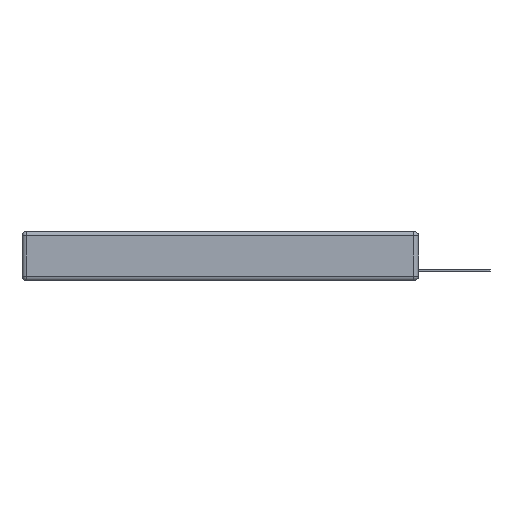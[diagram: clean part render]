
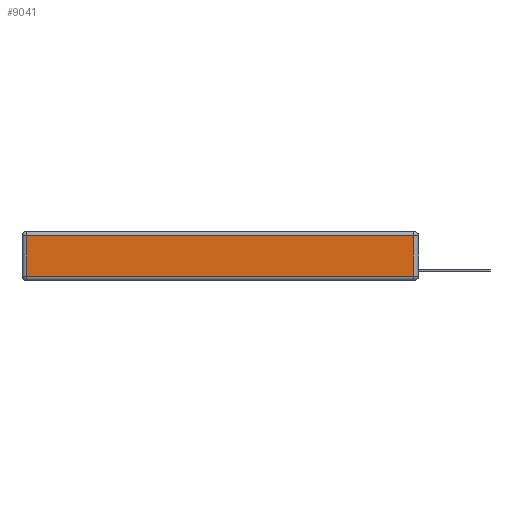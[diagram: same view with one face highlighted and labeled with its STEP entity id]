
A CAD part, left-side view. The second image highlights one B-rep face of the part: STEP entity #9041.
In plain terms, the highlighted planar face has unit normal (-1, 0, 0).
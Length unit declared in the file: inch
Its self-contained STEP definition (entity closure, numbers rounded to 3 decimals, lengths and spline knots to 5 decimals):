
#232 = EDGE_CURVE ( 'NONE', #12950, #11851, #2485, .T. ) ;
#245 = ORIENTED_EDGE ( 'NONE', *, *, #8034, .T. ) ;
#1006 = ORIENTED_EDGE ( 'NONE', *, *, #4992, .T. ) ;
#1263 = LINE ( 'NONE', #5545, #15086 ) ;
#1638 = DIRECTION ( 'NONE',  ( 0., 0., 1. ) ) ;
#2485 = LINE ( 'NONE', #7924, #13206 ) ;
#2680 = CARTESIAN_POINT ( 'NONE',  ( 0., 0.03, -0.313 ) ) ;
#3599 = VECTOR ( 'NONE', #1638, 39.37008 ) ;
#3632 = CARTESIAN_POINT ( 'NONE',  ( 0., 2.72, -0.03 ) ) ;
#4244 = CARTESIAN_POINT ( 'NONE',  ( 0., 2.72, -0.313 ) ) ;
#4803 = LINE ( 'NONE', #10966, #12752 ) ;
#4992 = EDGE_CURVE ( 'NONE', #8813, #12157, #4803, .T. ) ;
#4999 = CARTESIAN_POINT ( 'NONE',  ( 0., 0.03, -0.343 ) ) ;
#5394 = CARTESIAN_POINT ( 'NONE',  ( 0., 0.03, -0.03 ) ) ;
#5545 = CARTESIAN_POINT ( 'NONE',  ( 0., 2.72, -0.343 ) ) ;
#5698 = PLANE ( 'NONE',  #11499 ) ;
#5836 = LINE ( 'NONE', #4999, #3599 ) ;
#6877 = CARTESIAN_POINT ( 'NONE',  ( 0., 0., -0.343 ) ) ;
#7924 = CARTESIAN_POINT ( 'NONE',  ( 0., 2.75, -0.03 ) ) ;
#8034 = EDGE_CURVE ( 'NONE', #12157, #12950, #5836, .T. ) ;
#8718 = FACE_OUTER_BOUND ( 'NONE', #10525, .T. ) ;
#8813 = VERTEX_POINT ( 'NONE', #4244 ) ;
#9041 = ADVANCED_FACE ( 'NONE', ( #8718 ), #5698, .T. ) ;
#10252 = DIRECTION ( 'NONE',  ( 0., 0., -1. ) ) ;
#10482 = DIRECTION ( 'NONE',  ( 0., 0., 1. ) ) ;
#10525 = EDGE_LOOP ( 'NONE', ( #1006, #245, #13417, #14843 ) ) ;
#10966 = CARTESIAN_POINT ( 'NONE',  ( 0., 0., -0.313 ) ) ;
#11499 = AXIS2_PLACEMENT_3D ( 'NONE', #6877, #11743, #10482 ) ;
#11743 = DIRECTION ( 'NONE',  ( -1., 0., 0. ) ) ;
#11851 = VERTEX_POINT ( 'NONE', #3632 ) ;
#12157 = VERTEX_POINT ( 'NONE', #2680 ) ;
#12483 = DIRECTION ( 'NONE',  ( 0., 1., 0. ) ) ;
#12752 = VECTOR ( 'NONE', #14455, 39.37008 ) ;
#12950 = VERTEX_POINT ( 'NONE', #5394 ) ;
#13074 = EDGE_CURVE ( 'NONE', #11851, #8813, #1263, .T. ) ;
#13206 = VECTOR ( 'NONE', #12483, 39.37008 ) ;
#13417 = ORIENTED_EDGE ( 'NONE', *, *, #232, .T. ) ;
#14455 = DIRECTION ( 'NONE',  ( 0., -1., 0. ) ) ;
#14843 = ORIENTED_EDGE ( 'NONE', *, *, #13074, .T. ) ;
#15086 = VECTOR ( 'NONE', #10252, 39.37008 ) ;
